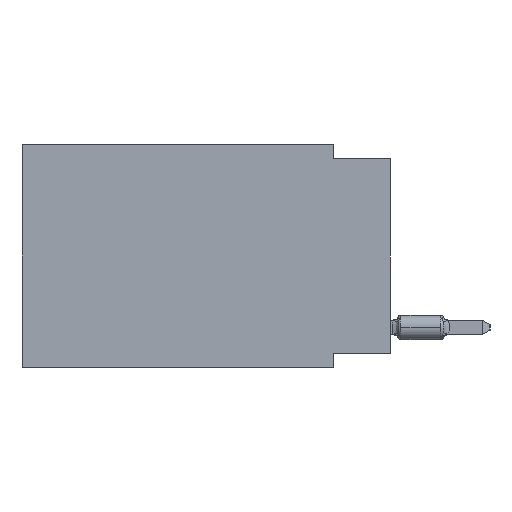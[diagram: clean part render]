
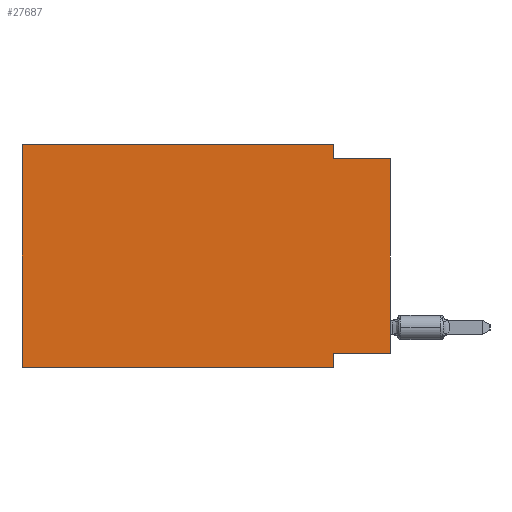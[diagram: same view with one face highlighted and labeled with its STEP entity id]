
A CAD part, left-side view. The second image highlights one B-rep face of the part: STEP entity #27687.
In plain terms, the highlighted planar face has unit normal (-1, 0, 0).
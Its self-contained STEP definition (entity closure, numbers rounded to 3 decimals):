
#201 = CARTESIAN_POINT ( 'NONE',  ( 0., 2.54, 0. ) ) ;
#275 = VECTOR ( 'NONE', #2008, 1000. ) ;
#346 = DIRECTION ( 'NONE',  ( 0., 0., -1. ) ) ;
#516 = VERTEX_POINT ( 'NONE', #14691 ) ;
#868 = LINE ( 'NONE', #7657, #25762 ) ;
#955 = VECTOR ( 'NONE', #13566, 1000. ) ;
#1143 = CARTESIAN_POINT ( 'NONE',  ( 0., 0., -9.271 ) ) ;
#1182 = CARTESIAN_POINT ( 'NONE',  ( 0., 2.54, -9.906 ) ) ;
#1968 = VERTEX_POINT ( 'NONE', #11585 ) ;
#2008 = DIRECTION ( 'NONE',  ( 0., -1., 0. ) ) ;
#3157 = VERTEX_POINT ( 'NONE', #1182 ) ;
#4001 = CARTESIAN_POINT ( 'NONE',  ( 0., 16.383, 0. ) ) ;
#4565 = CARTESIAN_POINT ( 'NONE',  ( 0., 2.54, 0. ) ) ;
#5068 = EDGE_CURVE ( 'NONE', #28065, #3157, #17856, .T. ) ;
#6009 = ORIENTED_EDGE ( 'NONE', *, *, #6103, .T. ) ;
#6029 = LINE ( 'NONE', #1143, #10111 ) ;
#6103 = EDGE_CURVE ( 'NONE', #516, #25353, #20367, .T. ) ;
#6372 = DIRECTION ( 'NONE',  ( 1., 0., 0. ) ) ;
#7057 = ORIENTED_EDGE ( 'NONE', *, *, #20300, .F. ) ;
#7657 = CARTESIAN_POINT ( 'NONE',  ( 0., 16.383, 0. ) ) ;
#9616 = CARTESIAN_POINT ( 'NONE',  ( 0., 16.383, 0. ) ) ;
#10045 = CARTESIAN_POINT ( 'NONE',  ( 0., 2.54, -9.271 ) ) ;
#10111 = VECTOR ( 'NONE', #21387, 1000. ) ;
#10278 = EDGE_LOOP ( 'NONE', ( #6009, #14580, #7057, #12502, #28307, #27597, #24220, #11457 ) ) ;
#11070 = CARTESIAN_POINT ( 'NONE',  ( 0., 16.383, 0. ) ) ;
#11336 = LINE ( 'NONE', #20337, #275 ) ;
#11457 = ORIENTED_EDGE ( 'NONE', *, *, #20035, .F. ) ;
#11585 = CARTESIAN_POINT ( 'NONE',  ( 0., 2.54, -0.635 ) ) ;
#12059 = CARTESIAN_POINT ( 'NONE',  ( 0., 2.54, -9.906 ) ) ;
#12502 = ORIENTED_EDGE ( 'NONE', *, *, #14695, .F. ) ;
#12946 = VECTOR ( 'NONE', #346, 1000. ) ;
#12976 = CARTESIAN_POINT ( 'NONE',  ( 0., 16.383, -9.906 ) ) ;
#13566 = DIRECTION ( 'NONE',  ( 0., -1., 0. ) ) ;
#13633 = VERTEX_POINT ( 'NONE', #10045 ) ;
#14580 = ORIENTED_EDGE ( 'NONE', *, *, #21541, .F. ) ;
#14691 = CARTESIAN_POINT ( 'NONE',  ( 0., 0., -9.271 ) ) ;
#14695 = EDGE_CURVE ( 'NONE', #21197, #19823, #868, .T. ) ;
#15215 = FACE_OUTER_BOUND ( 'NONE', #10278, .T. ) ;
#15500 = CARTESIAN_POINT ( 'NONE',  ( 0., 0., 0. ) ) ;
#15970 = EDGE_CURVE ( 'NONE', #28065, #21197, #20849, .T. ) ;
#16352 = VECTOR ( 'NONE', #18643, 1000. ) ;
#16628 = VECTOR ( 'NONE', #22453, 1000. ) ;
#17737 = EDGE_CURVE ( 'NONE', #13633, #3157, #18423, .T. ) ;
#17856 = LINE ( 'NONE', #29235, #955 ) ;
#18423 = LINE ( 'NONE', #12059, #24009 ) ;
#18563 = AXIS2_PLACEMENT_3D ( 'NONE', #4001, #6372, #22165 ) ;
#18643 = DIRECTION ( 'NONE',  ( 0., 0., 1. ) ) ;
#19823 = VERTEX_POINT ( 'NONE', #4565 ) ;
#20035 = EDGE_CURVE ( 'NONE', #516, #13633, #6029, .T. ) ;
#20300 = EDGE_CURVE ( 'NONE', #19823, #1968, #20444, .T. ) ;
#20337 = CARTESIAN_POINT ( 'NONE',  ( 0., 0., -0.635 ) ) ;
#20367 = LINE ( 'NONE', #15500, #16628 ) ;
#20444 = LINE ( 'NONE', #201, #12946 ) ;
#20849 = LINE ( 'NONE', #9616, #16352 ) ;
#21197 = VERTEX_POINT ( 'NONE', #11070 ) ;
#21387 = DIRECTION ( 'NONE',  ( 0., 1., 0. ) ) ;
#21541 = EDGE_CURVE ( 'NONE', #1968, #25353, #11336, .T. ) ;
#22165 = DIRECTION ( 'NONE',  ( 0., 0., -1. ) ) ;
#22453 = DIRECTION ( 'NONE',  ( 0., 0., 1. ) ) ;
#24009 = VECTOR ( 'NONE', #27734, 1000. ) ;
#24220 = ORIENTED_EDGE ( 'NONE', *, *, #17737, .F. ) ;
#24239 = PLANE ( 'NONE',  #18563 ) ;
#25353 = VERTEX_POINT ( 'NONE', #28374 ) ;
#25697 = DIRECTION ( 'NONE',  ( 0., -1., 0. ) ) ;
#25762 = VECTOR ( 'NONE', #25697, 1000. ) ;
#27597 = ORIENTED_EDGE ( 'NONE', *, *, #5068, .T. ) ;
#27687 = ADVANCED_FACE ( 'NONE', ( #15215 ), #24239, .F. ) ;
#27734 = DIRECTION ( 'NONE',  ( 0., 0., -1. ) ) ;
#28065 = VERTEX_POINT ( 'NONE', #12976 ) ;
#28307 = ORIENTED_EDGE ( 'NONE', *, *, #15970, .F. ) ;
#28374 = CARTESIAN_POINT ( 'NONE',  ( 0., 0., -0.635 ) ) ;
#29235 = CARTESIAN_POINT ( 'NONE',  ( 0., 16.383, -9.906 ) ) ;
